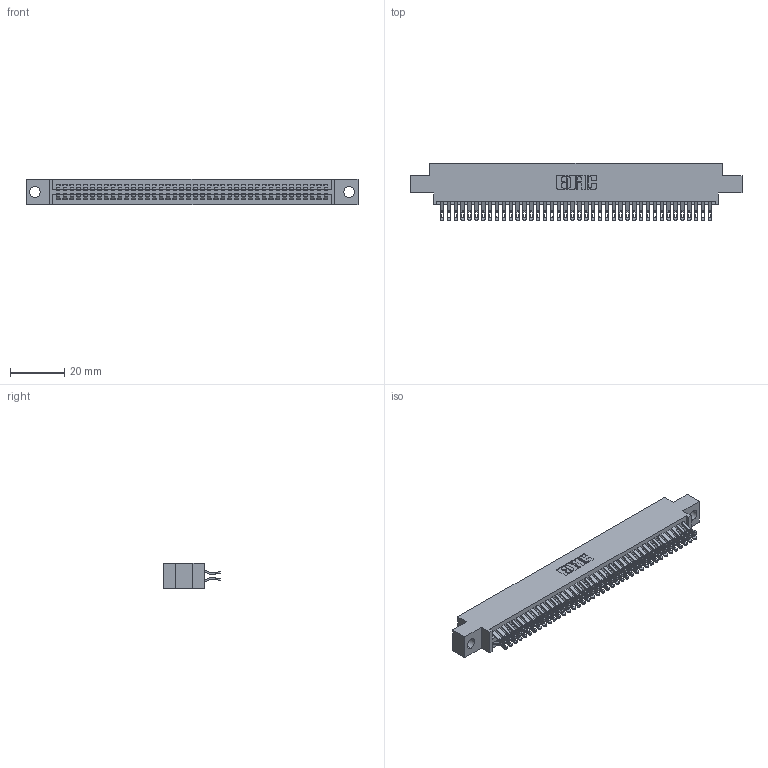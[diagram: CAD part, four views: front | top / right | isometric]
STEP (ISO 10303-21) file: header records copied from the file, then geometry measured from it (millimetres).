
FILE_DESCRIPTION (( 'STEP AP203' ), '1' );
FILE_NAME ('345-080-555-804.STEP', '2018-10-03T18:49:12', ( '' ), ( '' ), 'SwSTEP 2.0', 'SolidWorks 2016', '' );
FILE_SCHEMA (( 'CONFIG_CONTROL_DESIGN' ));
Length unit declared in the file: inch
Products named in the file (3): 345-080-555-804; 345 Part_0.170 Offset - 0.156 Dia-TH; 345-292-001_555 Tail
Assembly tree (81 placements, depth 2):
  345-080-555-804
    345 Part_0.170 Offset - 0.156 Dia-TH
    345-292-001_555 Tail  x80
Bounding box: 122.81 x 21.13 x 9.4 mm (x, y, z)
Volume: 11942 mm3; surface area: 18379.3 mm2
Topology: 81 solids, 81 shells, 4610 faces, 14513 edges, 9674 vertices
Faces by surface type: plane 2564, cylinder 2046
Entity records: 32115 total; most frequent: CARTESIAN_POINT 5422, ORIENTED_EDGE 5326, DIRECTION 4751, EDGE_CURVE 2663, VECTOR 2351, LINE 2351, VERTEX_POINT 1774, AXIS2_PLACEMENT_3D 1200
